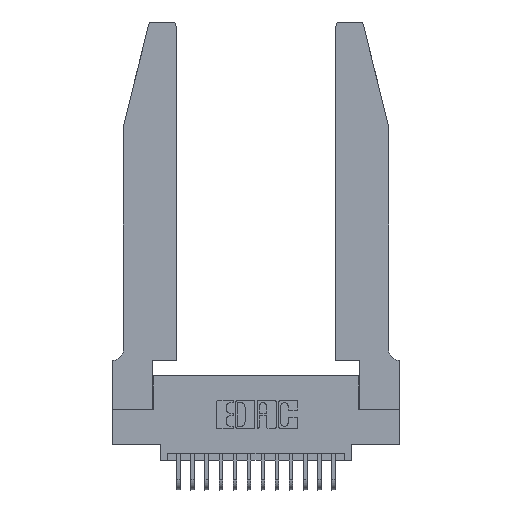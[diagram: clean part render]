
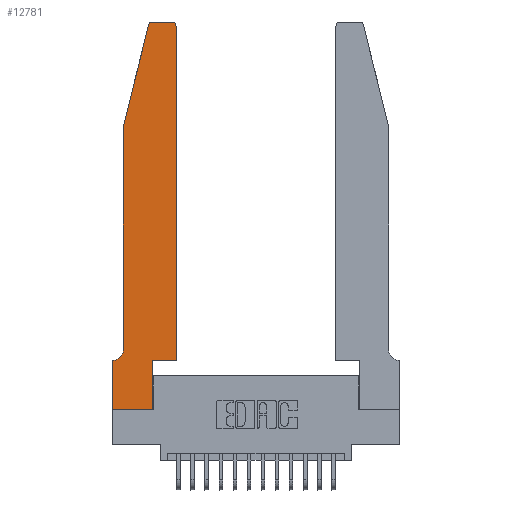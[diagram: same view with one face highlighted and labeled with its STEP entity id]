
A CAD part, top view. The second image highlights one B-rep face of the part: STEP entity #12781.
In plain terms, the highlighted planar face has unit normal (0, 0, 1).
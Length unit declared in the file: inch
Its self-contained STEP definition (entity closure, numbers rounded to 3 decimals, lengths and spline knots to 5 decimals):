
#4 = EDGE_CURVE ( 'NONE', #15360, #12561, #10790, .T. ) ;
#264 = CARTESIAN_POINT ( 'NONE',  ( 0.25487, 2.72718, 0.37 ) ) ;
#356 = VERTEX_POINT ( 'NONE', #6114 ) ;
#433 = DIRECTION ( 'NONE',  ( 1., 0., 0. ) ) ;
#682 = CIRCLE ( 'NONE', #16425, 0.03 ) ;
#954 = VERTEX_POINT ( 'NONE', #10950 ) ;
#1510 = EDGE_CURVE ( 'NONE', #7493, #8542, #9538, .T. ) ;
#1750 = CIRCLE ( 'NONE', #14297, 0.03 ) ;
#2003 = CARTESIAN_POINT ( 'NONE',  ( 0.0755, 2., 0.37 ) ) ;
#2437 = ORIENTED_EDGE ( 'NONE', *, *, #9895, .T. ) ;
#2545 = ORIENTED_EDGE ( 'NONE', *, *, #5563, .T. ) ;
#2888 = CARTESIAN_POINT ( 'NONE',  ( 0.0055, 0.35, 0.37 ) ) ;
#3120 = ORIENTED_EDGE ( 'NONE', *, *, #12044, .T. ) ;
#3377 = LINE ( 'NONE', #4186, #9416 ) ;
#3472 = ORIENTED_EDGE ( 'NONE', *, *, #4, .T. ) ;
#3655 = ORIENTED_EDGE ( 'NONE', *, *, #9268, .T. ) ;
#3782 = DIRECTION ( 'NONE',  ( 0., 0., 1. ) ) ;
#4186 = CARTESIAN_POINT ( 'NONE',  ( 0.0755, 2., 0.37 ) ) ;
#4819 = EDGE_CURVE ( 'NONE', #11949, #15360, #3377, .T. ) ;
#4959 = CARTESIAN_POINT ( 'NONE',  ( 0.0755, 0.35, 0.37 ) ) ;
#4997 = CARTESIAN_POINT ( 'NONE',  ( 0., 0., 0.37 ) ) ;
#5212 = EDGE_CURVE ( 'NONE', #12930, #8014, #13979, .T. ) ;
#5563 = EDGE_CURVE ( 'NONE', #8475, #11949, #682, .T. ) ;
#6114 = CARTESIAN_POINT ( 'NONE',  ( 0.4205, 2.75, 0.37 ) ) ;
#6808 = AXIS2_PLACEMENT_3D ( 'NONE', #17789, #14479, #8474 ) ;
#7493 = VERTEX_POINT ( 'NONE', #18734 ) ;
#7764 = ORIENTED_EDGE ( 'NONE', *, *, #17595, .T. ) ;
#8014 = VERTEX_POINT ( 'NONE', #13863 ) ;
#8035 = DIRECTION ( 'NONE',  ( -1., 0., 0. ) ) ;
#8083 = VECTOR ( 'NONE', #8727, 39.37008 ) ;
#8363 = CARTESIAN_POINT ( 'NONE',  ( 0.284, 2.72, 0.37 ) ) ;
#8474 = DIRECTION ( 'NONE',  ( 1., 0., 0. ) ) ;
#8475 = VERTEX_POINT ( 'NONE', #9029 ) ;
#8499 = CARTESIAN_POINT ( 'NONE',  ( 0.4205, 2.72, 0.37 ) ) ;
#8542 = VERTEX_POINT ( 'NONE', #16948 ) ;
#8555 = DIRECTION ( 'NONE',  ( 0., 0., 1. ) ) ;
#8678 = LINE ( 'NONE', #14355, #16188 ) ;
#8727 = DIRECTION ( 'NONE',  ( 0., 1., 0. ) ) ;
#9029 = CARTESIAN_POINT ( 'NONE',  ( 0.284, 2.75, 0.37 ) ) ;
#9268 = EDGE_CURVE ( 'NONE', #16328, #12930, #9726, .T. ) ;
#9416 = VECTOR ( 'NONE', #15683, 39.37008 ) ;
#9538 = LINE ( 'NONE', #16487, #8083 ) ;
#9626 = DIRECTION ( 'NONE',  ( -1., 0., 0. ) ) ;
#9726 = LINE ( 'NONE', #4959, #17478 ) ;
#9825 = VECTOR ( 'NONE', #10676, 39.37008 ) ;
#9867 = LINE ( 'NONE', #14451, #18576 ) ;
#9895 = EDGE_CURVE ( 'NONE', #13021, #356, #1750, .T. ) ;
#10159 = DIRECTION ( 'NONE',  ( 0., -1., 0. ) ) ;
#10589 = EDGE_CURVE ( 'NONE', #954, #13021, #18414, .T. ) ;
#10676 = DIRECTION ( 'NONE',  ( 0., -1., 0. ) ) ;
#10790 = LINE ( 'NONE', #15179, #9825 ) ;
#10950 = CARTESIAN_POINT ( 'NONE',  ( 0.4505, 0.35, 0.37 ) ) ;
#11338 = LINE ( 'NONE', #4997, #17846 ) ;
#11417 = DIRECTION ( 'NONE',  ( 1., 0., 0. ) ) ;
#11524 = ORIENTED_EDGE ( 'NONE', *, *, #5212, .T. ) ;
#11570 = ORIENTED_EDGE ( 'NONE', *, *, #10589, .T. ) ;
#11622 = ORIENTED_EDGE ( 'NONE', *, *, #4819, .T. ) ;
#11949 = VERTEX_POINT ( 'NONE', #264 ) ;
#11992 = CARTESIAN_POINT ( 'NONE',  ( 0.4505, 0.35, 0.37 ) ) ;
#12044 = EDGE_CURVE ( 'NONE', #8542, #954, #8678, .T. ) ;
#12127 = DIRECTION ( 'NONE',  ( 0., 1., 0. ) ) ;
#12554 = ORIENTED_EDGE ( 'NONE', *, *, #18226, .T. ) ;
#12561 = VERTEX_POINT ( 'NONE', #12874 ) ;
#12781 = ADVANCED_FACE ( 'NONE', ( #14456 ), #16173, .T. ) ;
#12874 = CARTESIAN_POINT ( 'NONE',  ( 0.0755, 0.42, 0.37 ) ) ;
#12930 = VERTEX_POINT ( 'NONE', #19550 ) ;
#13021 = VERTEX_POINT ( 'NONE', #13583 ) ;
#13328 = CIRCLE ( 'NONE', #18261, 0.07 ) ;
#13583 = CARTESIAN_POINT ( 'NONE',  ( 0.4505, 2.72, 0.37 ) ) ;
#13863 = CARTESIAN_POINT ( 'NONE',  ( 0., 0., 0.37 ) ) ;
#13979 = LINE ( 'NONE', #14591, #14947 ) ;
#14267 = VECTOR ( 'NONE', #12127, 39.37008 ) ;
#14297 = AXIS2_PLACEMENT_3D ( 'NONE', #8499, #8555, #11417 ) ;
#14355 = CARTESIAN_POINT ( 'NONE',  ( 0.4505, 0.35, 0.37 ) ) ;
#14451 = CARTESIAN_POINT ( 'NONE',  ( 0.2605, 2.75, 0.37 ) ) ;
#14456 = FACE_OUTER_BOUND ( 'NONE', #16295, .T. ) ;
#14479 = DIRECTION ( 'NONE',  ( 0., 0., 1. ) ) ;
#14569 = DIRECTION ( 'NONE',  ( 1., 0., 0. ) ) ;
#14591 = CARTESIAN_POINT ( 'NONE',  ( 0., 0., 0.37 ) ) ;
#14947 = VECTOR ( 'NONE', #10159, 39.37008 ) ;
#15179 = CARTESIAN_POINT ( 'NONE',  ( 0.0755, 2., 0.37 ) ) ;
#15360 = VERTEX_POINT ( 'NONE', #2003 ) ;
#15392 = DIRECTION ( 'NONE',  ( 0., 0., -1. ) ) ;
#15683 = DIRECTION ( 'NONE',  ( -0.239, -0.971, 0. ) ) ;
#15800 = EDGE_CURVE ( 'NONE', #12561, #16328, #13328, .T. ) ;
#16173 = PLANE ( 'NONE',  #6808 ) ;
#16188 = VECTOR ( 'NONE', #17426, 39.37008 ) ;
#16295 = EDGE_LOOP ( 'NONE', ( #12554, #2545, #11622, #3472, #18448, #3655, #11524, #7764, #18156, #3120, #11570, #2437 ) ) ;
#16328 = VERTEX_POINT ( 'NONE', #2888 ) ;
#16425 = AXIS2_PLACEMENT_3D ( 'NONE', #8363, #3782, #14569 ) ;
#16487 = CARTESIAN_POINT ( 'NONE',  ( 0.2865, 0.35, 0.37 ) ) ;
#16813 = CARTESIAN_POINT ( 'NONE',  ( 0.0055, 0.42, 0.37 ) ) ;
#16948 = CARTESIAN_POINT ( 'NONE',  ( 0.2865, 0.35, 0.37 ) ) ;
#17426 = DIRECTION ( 'NONE',  ( 1., 0., 0. ) ) ;
#17478 = VECTOR ( 'NONE', #9626, 39.37008 ) ;
#17595 = EDGE_CURVE ( 'NONE', #8014, #7493, #11338, .T. ) ;
#17789 = CARTESIAN_POINT ( 'NONE',  ( 0., 0.35, 0.37 ) ) ;
#17846 = VECTOR ( 'NONE', #433, 39.37008 ) ;
#18156 = ORIENTED_EDGE ( 'NONE', *, *, #1510, .T. ) ;
#18226 = EDGE_CURVE ( 'NONE', #356, #8475, #9867, .T. ) ;
#18261 = AXIS2_PLACEMENT_3D ( 'NONE', #16813, #15392, #18338 ) ;
#18338 = DIRECTION ( 'NONE',  ( -1., 0., 0. ) ) ;
#18414 = LINE ( 'NONE', #11992, #14267 ) ;
#18448 = ORIENTED_EDGE ( 'NONE', *, *, #15800, .T. ) ;
#18576 = VECTOR ( 'NONE', #8035, 39.37008 ) ;
#18734 = CARTESIAN_POINT ( 'NONE',  ( 0.2865, 0., 0.37 ) ) ;
#19550 = CARTESIAN_POINT ( 'NONE',  ( 0., 0.35, 0.37 ) ) ;
